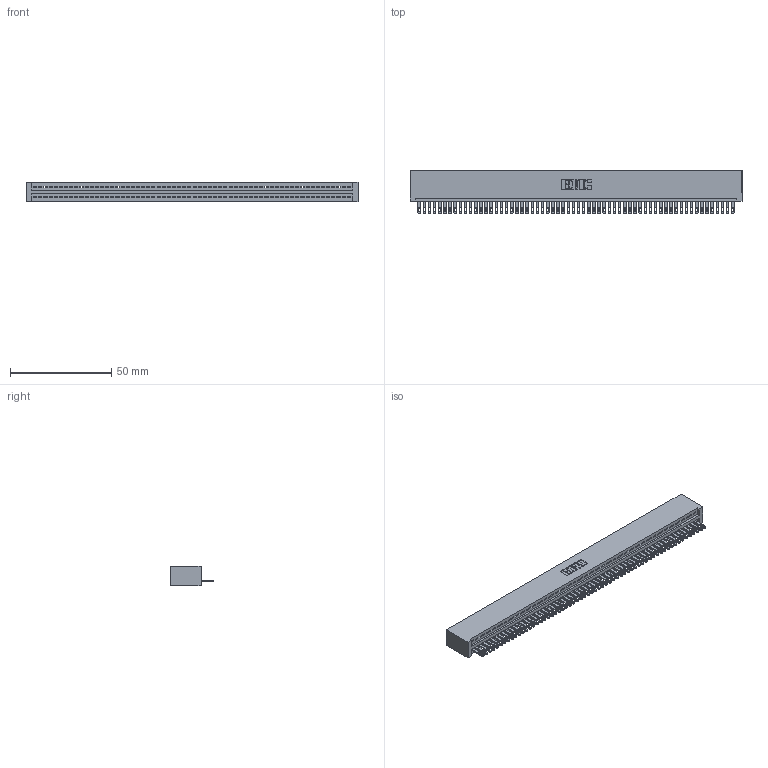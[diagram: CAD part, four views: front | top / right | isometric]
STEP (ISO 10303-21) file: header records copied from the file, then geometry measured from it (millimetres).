
FILE_DESCRIPTION (( 'STEP AP203' ), '1' );
FILE_NAME ('345-062-500-101.STEP', '2018-09-27T10:15:32', ( '' ), ( '' ), 'SwSTEP 2.0', 'SolidWorks 2016', '' );
FILE_SCHEMA (( 'CONFIG_CONTROL_DESIGN' ));
Length unit declared in the file: inch
Products named in the file (3): 345-292-001_345-293-100; 345-062-500-101; 345 Part_No Mounting Lugs
Assembly tree (63 placements, depth 2):
  345-062-500-101
    345 Part_No Mounting Lugs
    345-292-001_345-293-100  x62
Bounding box: 164.08 x 21.51 x 9.4 mm (x, y, z)
Volume: 16371.4 mm3; surface area: 22357.3 mm2
Topology: 63 solids, 63 shells, 3466 faces, 10733 edges, 7154 vertices
Faces by surface type: plane 2184, cylinder 1282
Entity records: 43623 total; most frequent: CARTESIAN_POINT 7562, ORIENTED_EDGE 7558, DIRECTION 6571, EDGE_CURVE 3779, LINE 3403, VECTOR 3403, VERTEX_POINT 2518, AXIS2_PLACEMENT_3D 1584
